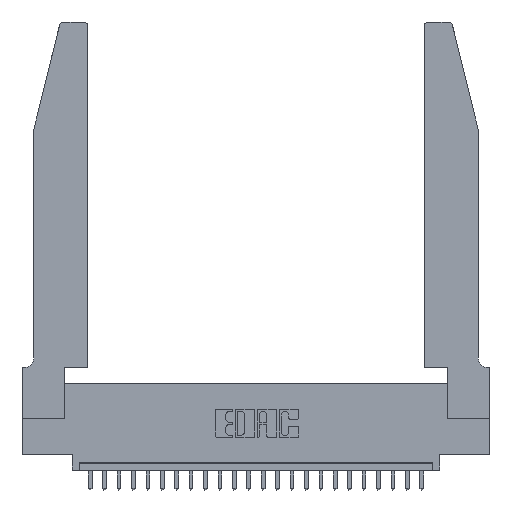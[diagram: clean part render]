
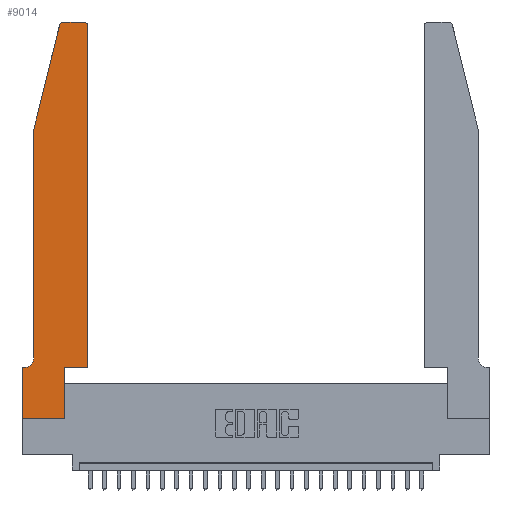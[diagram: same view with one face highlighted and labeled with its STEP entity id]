
A CAD part, top view. The second image highlights one B-rep face of the part: STEP entity #9014.
In plain terms, the highlighted planar face has unit normal (0, 0, 1).
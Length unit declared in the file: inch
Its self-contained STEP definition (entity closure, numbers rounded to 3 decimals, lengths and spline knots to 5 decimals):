
#151 = LINE ( 'NONE', #1384, #11208 ) ;
#255 = EDGE_CURVE ( 'NONE', #4184, #22375, #18025, .T. ) ;
#366 = CARTESIAN_POINT ( 'NONE',  ( 0.0055, 0.42, 0.37 ) ) ;
#371 = CARTESIAN_POINT ( 'NONE',  ( 0., 0., 0.37 ) ) ;
#395 = AXIS2_PLACEMENT_3D ( 'NONE', #24392, #16581, #8792 ) ;
#1020 = CARTESIAN_POINT ( 'NONE',  ( 0.4505, 0.35, 0.37 ) ) ;
#1384 = CARTESIAN_POINT ( 'NONE',  ( 0.0755, 2., 0.37 ) ) ;
#1535 = LINE ( 'NONE', #24013, #9802 ) ;
#1638 = ORIENTED_EDGE ( 'NONE', *, *, #18516, .T. ) ;
#1894 = LINE ( 'NONE', #1020, #12595 ) ;
#2079 = LINE ( 'NONE', #12252, #8528 ) ;
#2127 = ORIENTED_EDGE ( 'NONE', *, *, #8467, .T. ) ;
#2254 = VERTEX_POINT ( 'NONE', #19622 ) ;
#2276 = FACE_OUTER_BOUND ( 'NONE', #4364, .T. ) ;
#2704 = ORIENTED_EDGE ( 'NONE', *, *, #13514, .T. ) ;
#2770 = CARTESIAN_POINT ( 'NONE',  ( 0., 0.35, 0.37 ) ) ;
#3220 = VECTOR ( 'NONE', #24309, 39.37008 ) ;
#3314 = ORIENTED_EDGE ( 'NONE', *, *, #15313, .T. ) ;
#3483 = DIRECTION ( 'NONE',  ( 1., 0., 0. ) ) ;
#3499 = ORIENTED_EDGE ( 'NONE', *, *, #18445, .T. ) ;
#3550 = DIRECTION ( 'NONE',  ( -1., 0., 0. ) ) ;
#3613 = DIRECTION ( 'NONE',  ( 1., 0., 0. ) ) ;
#3968 = CIRCLE ( 'NONE', #15453, 0.03 ) ;
#4184 = VERTEX_POINT ( 'NONE', #24279 ) ;
#4364 = EDGE_LOOP ( 'NONE', ( #9920, #6720, #1638, #4889, #15587, #3499, #22964, #6398, #21080, #2704, #2127, #3314 ) ) ;
#4889 = ORIENTED_EDGE ( 'NONE', *, *, #20848, .T. ) ;
#5139 = LINE ( 'NONE', #371, #17380 ) ;
#5453 = CARTESIAN_POINT ( 'NONE',  ( 0.2605, 2.75, 0.37 ) ) ;
#6149 = DIRECTION ( 'NONE',  ( -0.239, -0.971, 0. ) ) ;
#6339 = LINE ( 'NONE', #22718, #10665 ) ;
#6398 = ORIENTED_EDGE ( 'NONE', *, *, #17217, .T. ) ;
#6399 = CARTESIAN_POINT ( 'NONE',  ( 0.2865, 0.35, 0.37 ) ) ;
#6401 = DIRECTION ( 'NONE',  ( -1., 0., 0. ) ) ;
#6573 = LINE ( 'NONE', #5453, #7468 ) ;
#6720 = ORIENTED_EDGE ( 'NONE', *, *, #255, .T. ) ;
#6835 = CARTESIAN_POINT ( 'NONE',  ( 0.4505, 0.35, 0.37 ) ) ;
#7468 = VECTOR ( 'NONE', #3550, 39.37008 ) ;
#8002 = CARTESIAN_POINT ( 'NONE',  ( 0.4505, 0.35, 0.37 ) ) ;
#8234 = DIRECTION ( 'NONE',  ( 0., 0., -1. ) ) ;
#8467 = EDGE_CURVE ( 'NONE', #17035, #19934, #19443, .T. ) ;
#8528 = VECTOR ( 'NONE', #6401, 39.37008 ) ;
#8792 = DIRECTION ( 'NONE',  ( 1., 0., 0. ) ) ;
#8874 = CARTESIAN_POINT ( 'NONE',  ( 0.0755, 2., 0.37 ) ) ;
#9014 = ADVANCED_FACE ( 'NONE', ( #2276 ), #9393, .T. ) ;
#9272 = EDGE_CURVE ( 'NONE', #23234, #4184, #6573, .T. ) ;
#9393 = PLANE ( 'NONE',  #22278 ) ;
#9789 = AXIS2_PLACEMENT_3D ( 'NONE', #366, #8234, #12392 ) ;
#9802 = VECTOR ( 'NONE', #18089, 39.37008 ) ;
#9920 = ORIENTED_EDGE ( 'NONE', *, *, #9272, .T. ) ;
#10665 = VECTOR ( 'NONE', #14857, 39.37008 ) ;
#11208 = VECTOR ( 'NONE', #22927, 39.37008 ) ;
#11934 = VECTOR ( 'NONE', #6149, 39.37008 ) ;
#12252 = CARTESIAN_POINT ( 'NONE',  ( 0.0755, 0.35, 0.37 ) ) ;
#12392 = DIRECTION ( 'NONE',  ( -1., 0., 0. ) ) ;
#12482 = VERTEX_POINT ( 'NONE', #18939 ) ;
#12595 = VECTOR ( 'NONE', #16418, 39.37008 ) ;
#12947 = VERTEX_POINT ( 'NONE', #21723 ) ;
#13509 = VERTEX_POINT ( 'NONE', #8874 ) ;
#13514 = EDGE_CURVE ( 'NONE', #23320, #17035, #1894, .T. ) ;
#14857 = DIRECTION ( 'NONE',  ( 0., 1., 0. ) ) ;
#15208 = CARTESIAN_POINT ( 'NONE',  ( 0., 0.35, 0.37 ) ) ;
#15297 = DIRECTION ( 'NONE',  ( 0., 0., 1. ) ) ;
#15313 = EDGE_CURVE ( 'NONE', #19934, #23234, #3968, .T. ) ;
#15453 = AXIS2_PLACEMENT_3D ( 'NONE', #18958, #25121, #3613 ) ;
#15587 = ORIENTED_EDGE ( 'NONE', *, *, #20656, .T. ) ;
#16418 = DIRECTION ( 'NONE',  ( 1., 0., 0. ) ) ;
#16581 = DIRECTION ( 'NONE',  ( 0., 0., 1. ) ) ;
#16987 = CIRCLE ( 'NONE', #9789, 0.07 ) ;
#17035 = VERTEX_POINT ( 'NONE', #8002 ) ;
#17079 = LINE ( 'NONE', #17856, #11934 ) ;
#17217 = EDGE_CURVE ( 'NONE', #12947, #12482, #1535, .T. ) ;
#17380 = VECTOR ( 'NONE', #24001, 39.37008 ) ;
#17454 = VERTEX_POINT ( 'NONE', #2770 ) ;
#17528 = CARTESIAN_POINT ( 'NONE',  ( 0.0755, 0.42, 0.37 ) ) ;
#17856 = CARTESIAN_POINT ( 'NONE',  ( 0.0755, 2., 0.37 ) ) ;
#18025 = CIRCLE ( 'NONE', #395, 0.03 ) ;
#18089 = DIRECTION ( 'NONE',  ( 1., 0., 0. ) ) ;
#18445 = EDGE_CURVE ( 'NONE', #2254, #17454, #2079, .T. ) ;
#18516 = EDGE_CURVE ( 'NONE', #22375, #13509, #17079, .T. ) ;
#18939 = CARTESIAN_POINT ( 'NONE',  ( 0.2865, 0., 0.37 ) ) ;
#18958 = CARTESIAN_POINT ( 'NONE',  ( 0.4205, 2.72, 0.37 ) ) ;
#19443 = LINE ( 'NONE', #6835, #3220 ) ;
#19622 = CARTESIAN_POINT ( 'NONE',  ( 0.0055, 0.35, 0.37 ) ) ;
#19742 = CARTESIAN_POINT ( 'NONE',  ( 0.4205, 2.75, 0.37 ) ) ;
#19872 = CARTESIAN_POINT ( 'NONE',  ( 0.25487, 2.72718, 0.37 ) ) ;
#19934 = VERTEX_POINT ( 'NONE', #20891 ) ;
#20656 = EDGE_CURVE ( 'NONE', #22826, #2254, #16987, .T. ) ;
#20848 = EDGE_CURVE ( 'NONE', #13509, #22826, #151, .T. ) ;
#20891 = CARTESIAN_POINT ( 'NONE',  ( 0.4505, 2.72, 0.37 ) ) ;
#21080 = ORIENTED_EDGE ( 'NONE', *, *, #25200, .T. ) ;
#21723 = CARTESIAN_POINT ( 'NONE',  ( 0., 0., 0.37 ) ) ;
#22278 = AXIS2_PLACEMENT_3D ( 'NONE', #15208, #15297, #3483 ) ;
#22375 = VERTEX_POINT ( 'NONE', #19872 ) ;
#22718 = CARTESIAN_POINT ( 'NONE',  ( 0.2865, 0.35, 0.37 ) ) ;
#22826 = VERTEX_POINT ( 'NONE', #17528 ) ;
#22927 = DIRECTION ( 'NONE',  ( 0., -1., 0. ) ) ;
#22964 = ORIENTED_EDGE ( 'NONE', *, *, #23803, .T. ) ;
#23234 = VERTEX_POINT ( 'NONE', #19742 ) ;
#23320 = VERTEX_POINT ( 'NONE', #6399 ) ;
#23803 = EDGE_CURVE ( 'NONE', #17454, #12947, #5139, .T. ) ;
#24001 = DIRECTION ( 'NONE',  ( 0., -1., 0. ) ) ;
#24013 = CARTESIAN_POINT ( 'NONE',  ( 0., 0., 0.37 ) ) ;
#24279 = CARTESIAN_POINT ( 'NONE',  ( 0.284, 2.75, 0.37 ) ) ;
#24309 = DIRECTION ( 'NONE',  ( 0., 1., 0. ) ) ;
#24392 = CARTESIAN_POINT ( 'NONE',  ( 0.284, 2.72, 0.37 ) ) ;
#25121 = DIRECTION ( 'NONE',  ( 0., 0., 1. ) ) ;
#25200 = EDGE_CURVE ( 'NONE', #12482, #23320, #6339, .T. ) ;
